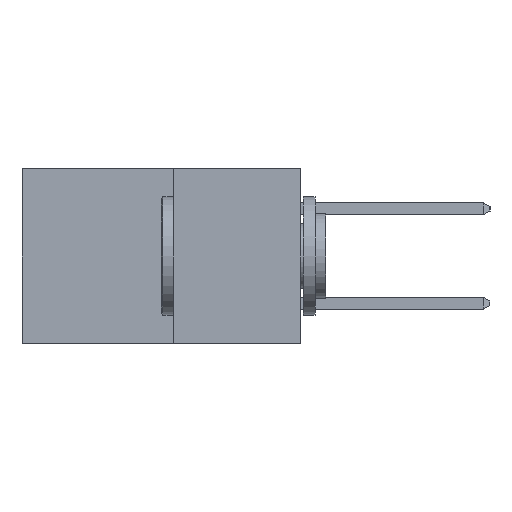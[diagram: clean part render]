
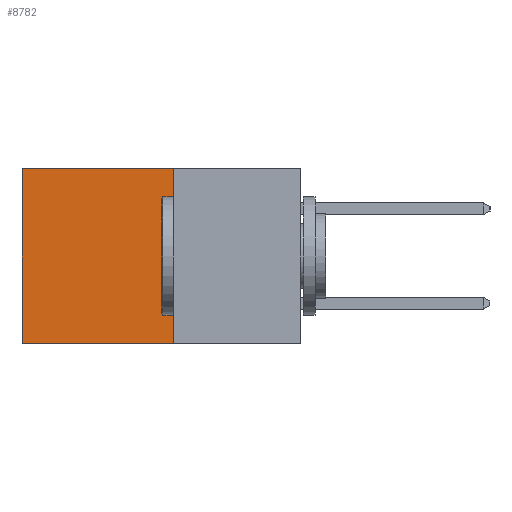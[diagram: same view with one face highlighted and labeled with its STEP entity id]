
A CAD part, left-side view. The second image highlights one B-rep face of the part: STEP entity #8782.
In plain terms, the highlighted planar face has unit normal (-1, 0, 0).
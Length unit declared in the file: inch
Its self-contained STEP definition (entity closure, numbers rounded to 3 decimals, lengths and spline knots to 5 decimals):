
#644 = LINE ( 'NONE', #18981, #15573 ) ;
#1348 = EDGE_CURVE ( 'NONE', #23326, #6507, #644, .T. ) ;
#4720 = DIRECTION ( 'NONE',  ( 1., 0., 0. ) ) ;
#4974 = CARTESIAN_POINT ( 'NONE',  ( 0.277, 0.27, 0. ) ) ;
#5021 = EDGE_CURVE ( 'NONE', #5529, #6507, #23776, .T. ) ;
#5134 = CARTESIAN_POINT ( 'NONE',  ( 0.277, 0.27, -0.37 ) ) ;
#5245 = DIRECTION ( 'NONE',  ( 0., 0., -1. ) ) ;
#5529 = VERTEX_POINT ( 'NONE', #13069 ) ;
#5658 = AXIS2_PLACEMENT_3D ( 'NONE', #10477, #4720, #18285 ) ;
#6507 = VERTEX_POINT ( 'NONE', #7873 ) ;
#7873 = CARTESIAN_POINT ( 'NONE',  ( 0.277, 0.59, -0.37 ) ) ;
#8621 = ORIENTED_EDGE ( 'NONE', *, *, #17401, .T. ) ;
#8782 = ADVANCED_FACE ( 'NONE', ( #9166 ), #16349, .F. ) ;
#8850 = VERTEX_POINT ( 'NONE', #4974 ) ;
#9127 = ORIENTED_EDGE ( 'NONE', *, *, #14258, .F. ) ;
#9166 = FACE_OUTER_BOUND ( 'NONE', #20821, .T. ) ;
#9181 = LINE ( 'NONE', #16090, #18908 ) ;
#10192 = VECTOR ( 'NONE', #5245, 39.37008 ) ;
#10477 = CARTESIAN_POINT ( 'NONE',  ( 0.277, 0.27, -0.37 ) ) ;
#13069 = CARTESIAN_POINT ( 'NONE',  ( 0.277, 0.59, 0. ) ) ;
#13550 = LINE ( 'NONE', #22668, #10192 ) ;
#13578 = VECTOR ( 'NONE', #20541, 39.37008 ) ;
#13761 = ORIENTED_EDGE ( 'NONE', *, *, #1348, .F. ) ;
#14258 = EDGE_CURVE ( 'NONE', #8850, #23326, #13550, .T. ) ;
#15573 = VECTOR ( 'NONE', #19288, 39.37008 ) ;
#16090 = CARTESIAN_POINT ( 'NONE',  ( 0.277, 0.27, 0. ) ) ;
#16349 = PLANE ( 'NONE',  #5658 ) ;
#17316 = ORIENTED_EDGE ( 'NONE', *, *, #5021, .T. ) ;
#17401 = EDGE_CURVE ( 'NONE', #8850, #5529, #9181, .T. ) ;
#18033 = DIRECTION ( 'NONE',  ( 0., 1., 0. ) ) ;
#18285 = DIRECTION ( 'NONE',  ( 0., 0., -1. ) ) ;
#18908 = VECTOR ( 'NONE', #18033, 39.37008 ) ;
#18981 = CARTESIAN_POINT ( 'NONE',  ( 0.277, 0.27, -0.37 ) ) ;
#19288 = DIRECTION ( 'NONE',  ( 0., 1., 0. ) ) ;
#20311 = CARTESIAN_POINT ( 'NONE',  ( 0.277, 0.59, -0.37 ) ) ;
#20541 = DIRECTION ( 'NONE',  ( 0., 0., -1. ) ) ;
#20821 = EDGE_LOOP ( 'NONE', ( #17316, #13761, #9127, #8621 ) ) ;
#22668 = CARTESIAN_POINT ( 'NONE',  ( 0.277, 0.27, -0.37 ) ) ;
#23326 = VERTEX_POINT ( 'NONE', #5134 ) ;
#23776 = LINE ( 'NONE', #20311, #13578 ) ;
